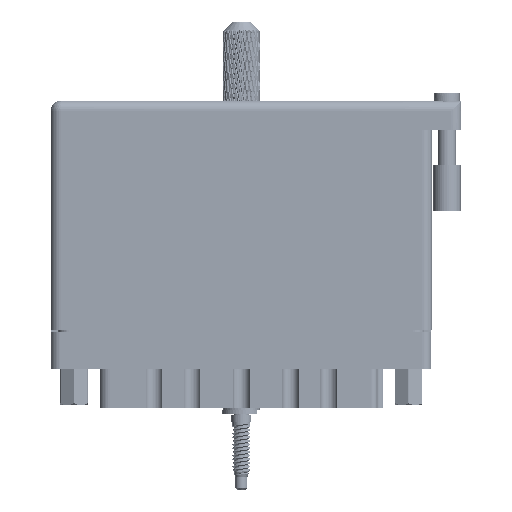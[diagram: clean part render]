
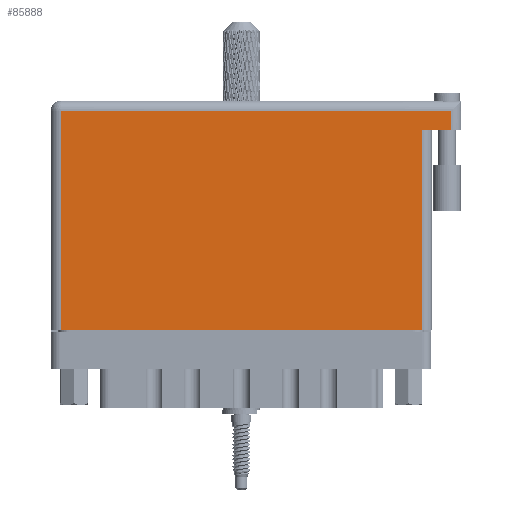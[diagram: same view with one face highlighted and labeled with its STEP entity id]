
A CAD part, front view. The second image highlights one B-rep face of the part: STEP entity #85888.
In plain terms, the highlighted face is planar.
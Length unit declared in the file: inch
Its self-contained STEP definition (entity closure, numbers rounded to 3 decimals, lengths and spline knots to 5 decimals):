
#377 = EDGE_CURVE ( 'NONE', #76233, #8145, #54234, .T. ) ;
#1676 = EDGE_LOOP ( 'NONE', ( #49264, #68296, #118752, #58740, #44300, #8321 ) ) ;
#6249 = CARTESIAN_POINT ( 'NONE',  ( 2.53, 0., 0. ) ) ;
#8145 = VERTEX_POINT ( 'NONE', #94431 ) ;
#8321 = ORIENTED_EDGE ( 'NONE', *, *, #377, .T. ) ;
#11120 = EDGE_CURVE ( 'NONE', #14012, #18178, #118977, .T. ) ;
#11553 = EDGE_CURVE ( 'NONE', #86594, #18178, #71186, .T. ) ;
#12971 = CARTESIAN_POINT ( 'NONE',  ( 0., 0., 0. ) ) ;
#13815 = CARTESIAN_POINT ( 'NONE',  ( 2.73, 1.496, 0. ) ) ;
#14012 = VERTEX_POINT ( 'NONE', #42747 ) ;
#14391 = DIRECTION ( 'NONE',  ( -1., 0., 0. ) ) ;
#14660 = VECTOR ( 'NONE', #25879, 39.37008 ) ;
#16841 = LINE ( 'NONE', #12971, #89372 ) ;
#18178 = VERTEX_POINT ( 'NONE', #57049 ) ;
#21791 = VECTOR ( 'NONE', #70719, 39.37008 ) ;
#25879 = DIRECTION ( 'NONE',  ( 0., 1., 0. ) ) ;
#26317 = VECTOR ( 'NONE', #112047, 39.37008 ) ;
#27488 = EDGE_CURVE ( 'NONE', #58321, #76233, #66636, .T. ) ;
#36071 = FACE_OUTER_BOUND ( 'NONE', #1676, .T. ) ;
#37102 = CARTESIAN_POINT ( 'NONE',  ( 2.73, 1.566, 0. ) ) ;
#41790 = VECTOR ( 'NONE', #67316, 39.37008 ) ;
#42747 = CARTESIAN_POINT ( 'NONE',  ( 2.73, 1.369, 0. ) ) ;
#44300 = ORIENTED_EDGE ( 'NONE', *, *, #27488, .T. ) ;
#49264 = ORIENTED_EDGE ( 'NONE', *, *, #57044, .T. ) ;
#51870 = DIRECTION ( 'NONE',  ( 0., 0., -1. ) ) ;
#53444 = DIRECTION ( 'NONE',  ( 1., 0., 0. ) ) ;
#54234 = LINE ( 'NONE', #78957, #21791 ) ;
#57044 = EDGE_CURVE ( 'NONE', #8145, #86594, #16841, .T. ) ;
#57049 = CARTESIAN_POINT ( 'NONE',  ( 2.53, 1.369, 0. ) ) ;
#58321 = VERTEX_POINT ( 'NONE', #13815 ) ;
#58740 = ORIENTED_EDGE ( 'NONE', *, *, #61579, .T. ) ;
#61329 = CARTESIAN_POINT ( 'NONE',  ( 0.07, 1.496, 0. ) ) ;
#61579 = EDGE_CURVE ( 'NONE', #14012, #58321, #102654, .T. ) ;
#66636 = LINE ( 'NONE', #126362, #41790 ) ;
#67316 = DIRECTION ( 'NONE',  ( -1., 0., 0. ) ) ;
#68296 = ORIENTED_EDGE ( 'NONE', *, *, #11553, .T. ) ;
#70719 = DIRECTION ( 'NONE',  ( 0., -1., 0. ) ) ;
#71186 = LINE ( 'NONE', #101794, #26317 ) ;
#73038 = DIRECTION ( 'NONE',  ( -1., 0., 0. ) ) ;
#76233 = VERTEX_POINT ( 'NONE', #61329 ) ;
#78957 = CARTESIAN_POINT ( 'NONE',  ( 0.07, 0., 0. ) ) ;
#79463 = AXIS2_PLACEMENT_3D ( 'NONE', #121708, #51870, #14391 ) ;
#85888 = ADVANCED_FACE ( 'NONE', ( #36071 ), #102817, .F. ) ;
#86594 = VERTEX_POINT ( 'NONE', #6249 ) ;
#89372 = VECTOR ( 'NONE', #53444, 39.37008 ) ;
#94431 = CARTESIAN_POINT ( 'NONE',  ( 0.07, 0., 0. ) ) ;
#101794 = CARTESIAN_POINT ( 'NONE',  ( 2.53, 1.369, 0. ) ) ;
#102654 = LINE ( 'NONE', #37102, #14660 ) ;
#102817 = PLANE ( 'NONE',  #79463 ) ;
#112047 = DIRECTION ( 'NONE',  ( 0., 1., 0. ) ) ;
#117522 = VECTOR ( 'NONE', #73038, 39.37008 ) ;
#118752 = ORIENTED_EDGE ( 'NONE', *, *, #11120, .F. ) ;
#118977 = LINE ( 'NONE', #122944, #117522 ) ;
#121708 = CARTESIAN_POINT ( 'NONE',  ( 0., 1.566, 0. ) ) ;
#122944 = CARTESIAN_POINT ( 'NONE',  ( 2.8, 1.369, 0. ) ) ;
#126362 = CARTESIAN_POINT ( 'NONE',  ( 0., 1.496, 0. ) ) ;
